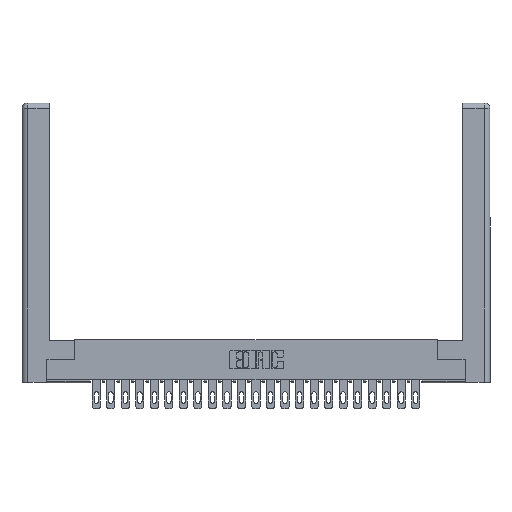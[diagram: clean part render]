
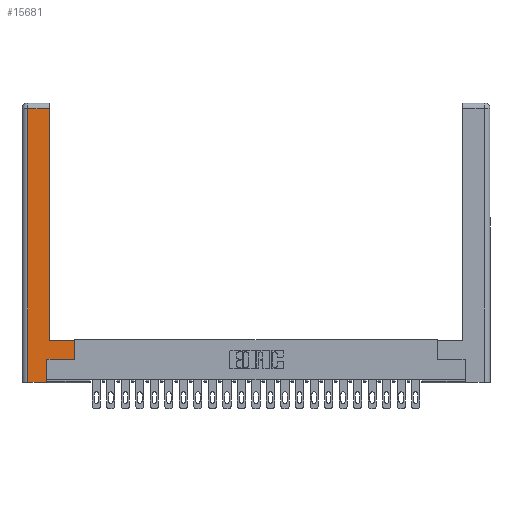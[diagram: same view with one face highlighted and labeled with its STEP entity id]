
A CAD part, top view. The second image highlights one B-rep face of the part: STEP entity #15681.
In plain terms, the highlighted planar face has unit normal (0, 0, 1).
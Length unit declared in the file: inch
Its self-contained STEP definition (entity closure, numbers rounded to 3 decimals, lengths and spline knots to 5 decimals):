
#1677 = CARTESIAN_POINT ( 'NONE',  ( 0.265, 0., 0. ) ) ;
#1826 = EDGE_CURVE ( 'NONE', #8316, #16170, #3753, .T. ) ;
#2141 = VECTOR ( 'NONE', #8922, 39.37008 ) ;
#2143 = VECTOR ( 'NONE', #18636, 39.37008 ) ;
#2591 = VERTEX_POINT ( 'NONE', #20421 ) ;
#3306 = VERTEX_POINT ( 'NONE', #13609 ) ;
#3753 = LINE ( 'NONE', #22667, #11979 ) ;
#4766 = VERTEX_POINT ( 'NONE', #24682 ) ;
#5283 = PLANE ( 'NONE',  #19393 ) ;
#5299 = VERTEX_POINT ( 'NONE', #1677 ) ;
#5331 = VECTOR ( 'NONE', #20636, 39.37008 ) ;
#5440 = ORIENTED_EDGE ( 'NONE', *, *, #1826, .T. ) ;
#6106 = EDGE_LOOP ( 'NONE', ( #5440, #9272, #18372, #14085, #20338, #9083, #26053, #24900 ) ) ;
#6273 = CARTESIAN_POINT ( 'NONE',  ( 0.565, 0.245, 0. ) ) ;
#6751 = CARTESIAN_POINT ( 'NONE',  ( 0.265, 0.245, 0. ) ) ;
#7126 = VERTEX_POINT ( 'NONE', #20434 ) ;
#7318 = DIRECTION ( 'NONE',  ( -1., 0., 0. ) ) ;
#8316 = VERTEX_POINT ( 'NONE', #9669 ) ;
#8366 = VERTEX_POINT ( 'NONE', #24395 ) ;
#8383 = LINE ( 'NONE', #20821, #25234 ) ;
#8634 = CARTESIAN_POINT ( 'NONE',  ( 0.265, 0., 0. ) ) ;
#8922 = DIRECTION ( 'NONE',  ( 0., 1., 0. ) ) ;
#9083 = ORIENTED_EDGE ( 'NONE', *, *, #15021, .T. ) ;
#9272 = ORIENTED_EDGE ( 'NONE', *, *, #12869, .T. ) ;
#9669 = CARTESIAN_POINT ( 'NONE',  ( 0.295, 0.45, 0. ) ) ;
#10484 = LINE ( 'NONE', #6273, #16928 ) ;
#11188 = LINE ( 'NONE', #8634, #18133 ) ;
#11919 = CARTESIAN_POINT ( 'NONE',  ( 0.0615, 2.94, 0. ) ) ;
#11979 = VECTOR ( 'NONE', #12005, 39.37008 ) ;
#12005 = DIRECTION ( 'NONE',  ( 0., 1., 0. ) ) ;
#12112 = VECTOR ( 'NONE', #26494, 39.37008 ) ;
#12869 = EDGE_CURVE ( 'NONE', #16170, #4766, #20148, .T. ) ;
#13609 = CARTESIAN_POINT ( 'NONE',  ( 0.565, 0.45, 0. ) ) ;
#14085 = ORIENTED_EDGE ( 'NONE', *, *, #23137, .T. ) ;
#14446 = CARTESIAN_POINT ( 'NONE',  ( 0.295, 0.45, 0. ) ) ;
#15021 = EDGE_CURVE ( 'NONE', #2591, #7126, #10484, .T. ) ;
#15681 = ADVANCED_FACE ( 'NONE', ( #23817 ), #5283, .F. ) ;
#16071 = CARTESIAN_POINT ( 'NONE',  ( 0.295, 2.94, 0. ) ) ;
#16160 = EDGE_CURVE ( 'NONE', #4766, #8366, #26336, .T. ) ;
#16170 = VERTEX_POINT ( 'NONE', #16071 ) ;
#16634 = DIRECTION ( 'NONE',  ( 0., 1., 0. ) ) ;
#16928 = VECTOR ( 'NONE', #18710, 39.37008 ) ;
#17063 = EDGE_CURVE ( 'NONE', #7126, #3306, #8383, .T. ) ;
#18133 = VECTOR ( 'NONE', #25119, 39.37008 ) ;
#18372 = ORIENTED_EDGE ( 'NONE', *, *, #16160, .T. ) ;
#18636 = DIRECTION ( 'NONE',  ( -1., 0., 0. ) ) ;
#18710 = DIRECTION ( 'NONE',  ( 1., 0., 0. ) ) ;
#18888 = LINE ( 'NONE', #14446, #2143 ) ;
#19310 = EDGE_CURVE ( 'NONE', #5299, #2591, #25270, .T. ) ;
#19393 = AXIS2_PLACEMENT_3D ( 'NONE', #19881, #24225, #7318 ) ;
#19881 = CARTESIAN_POINT ( 'NONE',  ( 0., 0., 0. ) ) ;
#20148 = LINE ( 'NONE', #11919, #12112 ) ;
#20338 = ORIENTED_EDGE ( 'NONE', *, *, #19310, .T. ) ;
#20421 = CARTESIAN_POINT ( 'NONE',  ( 0.265, 0.245, 0. ) ) ;
#20434 = CARTESIAN_POINT ( 'NONE',  ( 0.565, 0.245, 0. ) ) ;
#20636 = DIRECTION ( 'NONE',  ( 0., -1., 0. ) ) ;
#20821 = CARTESIAN_POINT ( 'NONE',  ( 0.565, 0.45, 0. ) ) ;
#22667 = CARTESIAN_POINT ( 'NONE',  ( 0.295, 3., 0. ) ) ;
#23137 = EDGE_CURVE ( 'NONE', #8366, #5299, #11188, .T. ) ;
#23817 = FACE_OUTER_BOUND ( 'NONE', #6106, .T. ) ;
#24225 = DIRECTION ( 'NONE',  ( 0., 0., -1. ) ) ;
#24311 = CARTESIAN_POINT ( 'NONE',  ( 0.0615, 0., 0. ) ) ;
#24347 = EDGE_CURVE ( 'NONE', #3306, #8316, #18888, .T. ) ;
#24395 = CARTESIAN_POINT ( 'NONE',  ( 0.0615, 0., 0. ) ) ;
#24682 = CARTESIAN_POINT ( 'NONE',  ( 0.0615, 2.94, 0. ) ) ;
#24900 = ORIENTED_EDGE ( 'NONE', *, *, #24347, .T. ) ;
#25119 = DIRECTION ( 'NONE',  ( 1., 0., 0. ) ) ;
#25234 = VECTOR ( 'NONE', #16634, 39.37008 ) ;
#25270 = LINE ( 'NONE', #6751, #2141 ) ;
#26053 = ORIENTED_EDGE ( 'NONE', *, *, #17063, .T. ) ;
#26336 = LINE ( 'NONE', #24311, #5331 ) ;
#26494 = DIRECTION ( 'NONE',  ( -1., 0., 0. ) ) ;
